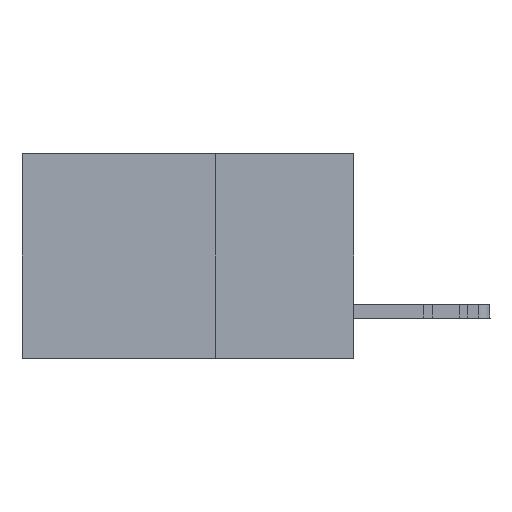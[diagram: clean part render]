
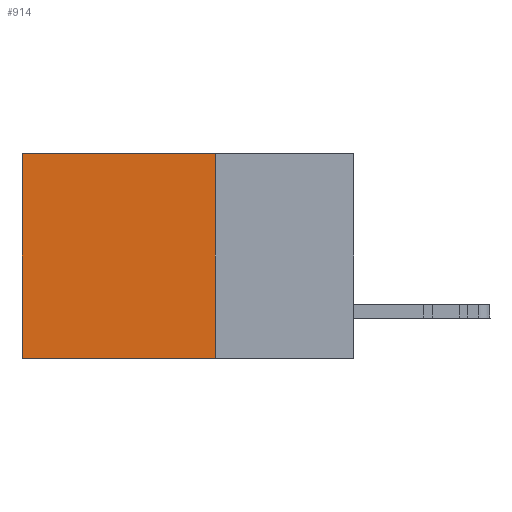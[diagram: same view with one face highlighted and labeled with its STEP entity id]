
A CAD part, left-side view. The second image highlights one B-rep face of the part: STEP entity #914.
In plain terms, the highlighted planar face has unit normal (-1, 0, 0).
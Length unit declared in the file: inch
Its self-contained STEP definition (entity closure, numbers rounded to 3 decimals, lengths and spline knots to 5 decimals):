
#10 = VECTOR ( 'NONE', #13287, 39.37008 ) ;
#226 = CARTESIAN_POINT ( 'NONE',  ( 0.2875, 0.25, 0. ) ) ;
#914 = ADVANCED_FACE ( 'NONE', ( #20206 ), #36616, .F. ) ;
#3150 = LINE ( 'NONE', #25695, #35443 ) ;
#4773 = LINE ( 'NONE', #33212, #34334 ) ;
#5384 = ORIENTED_EDGE ( 'NONE', *, *, #47435, .F. ) ;
#6026 = DIRECTION ( 'NONE',  ( 0., 1., 0. ) ) ;
#8712 = EDGE_CURVE ( 'NONE', #11866, #15719, #13341, .T. ) ;
#11249 = DIRECTION ( 'NONE',  ( 0., 0., -1. ) ) ;
#11866 = VERTEX_POINT ( 'NONE', #26023 ) ;
#12535 = CARTESIAN_POINT ( 'NONE',  ( 0.2875, 0.25, -0.37 ) ) ;
#12574 = ORIENTED_EDGE ( 'NONE', *, *, #43265, .F. ) ;
#13287 = DIRECTION ( 'NONE',  ( 0., 1., 0. ) ) ;
#13341 = LINE ( 'NONE', #41783, #27684 ) ;
#13962 = DIRECTION ( 'NONE',  ( 0., 0., -1. ) ) ;
#15574 = EDGE_LOOP ( 'NONE', ( #42061, #12574, #5384, #17093 ) ) ;
#15719 = VERTEX_POINT ( 'NONE', #39015 ) ;
#15771 = CARTESIAN_POINT ( 'NONE',  ( 0.2875, 0.25, -0.37 ) ) ;
#17093 = ORIENTED_EDGE ( 'NONE', *, *, #47828, .T. ) ;
#19299 = VERTEX_POINT ( 'NONE', #226 ) ;
#20206 = FACE_OUTER_BOUND ( 'NONE', #15574, .T. ) ;
#25695 = CARTESIAN_POINT ( 'NONE',  ( 0.2875, 0.25, 0. ) ) ;
#26023 = CARTESIAN_POINT ( 'NONE',  ( 0.2875, 0.6, 0. ) ) ;
#27684 = VECTOR ( 'NONE', #11249, 39.37008 ) ;
#29135 = CARTESIAN_POINT ( 'NONE',  ( 0.2875, 0.25, 0. ) ) ;
#33212 = CARTESIAN_POINT ( 'NONE',  ( 0.2875, 0.25, 0. ) ) ;
#34334 = VECTOR ( 'NONE', #6026, 39.37008 ) ;
#35340 = AXIS2_PLACEMENT_3D ( 'NONE', #29135, #47246, #13962 ) ;
#35443 = VECTOR ( 'NONE', #37570, 39.37008 ) ;
#36616 = PLANE ( 'NONE',  #35340 ) ;
#37570 = DIRECTION ( 'NONE',  ( 0., 0., -1. ) ) ;
#39015 = CARTESIAN_POINT ( 'NONE',  ( 0.2875, 0.6, -0.37 ) ) ;
#41783 = CARTESIAN_POINT ( 'NONE',  ( 0.2875, 0.6, 0. ) ) ;
#41850 = VERTEX_POINT ( 'NONE', #12535 ) ;
#42061 = ORIENTED_EDGE ( 'NONE', *, *, #8712, .T. ) ;
#43265 = EDGE_CURVE ( 'NONE', #41850, #15719, #49000, .T. ) ;
#47246 = DIRECTION ( 'NONE',  ( 1., 0., 0. ) ) ;
#47435 = EDGE_CURVE ( 'NONE', #19299, #41850, #3150, .T. ) ;
#47828 = EDGE_CURVE ( 'NONE', #19299, #11866, #4773, .T. ) ;
#49000 = LINE ( 'NONE', #15771, #10 ) ;
